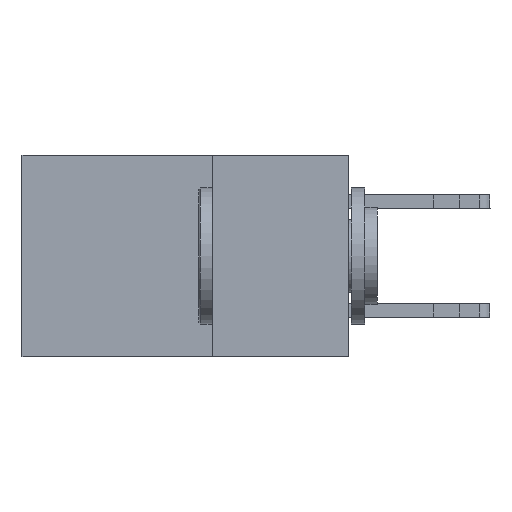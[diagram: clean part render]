
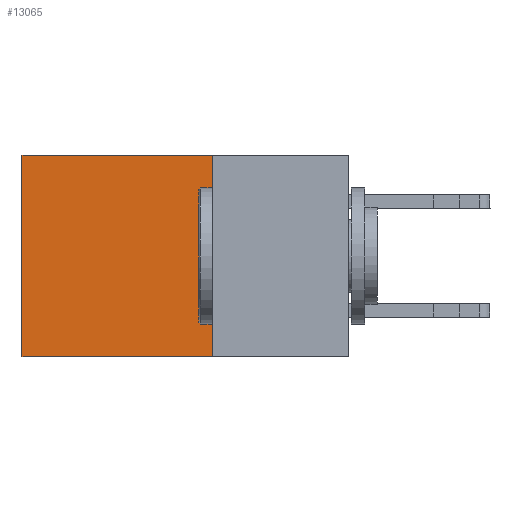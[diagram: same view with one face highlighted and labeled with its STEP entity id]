
A CAD part, left-side view. The second image highlights one B-rep face of the part: STEP entity #13065.
In plain terms, the highlighted planar face has unit normal (-1, 0, 0).
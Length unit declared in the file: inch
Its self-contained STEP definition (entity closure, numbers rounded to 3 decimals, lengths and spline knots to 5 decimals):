
#468 = DIRECTION ( 'NONE',  ( 1., 0., 0. ) ) ;
#1543 = LINE ( 'NONE', #2800, #16800 ) ;
#1731 = ORIENTED_EDGE ( 'NONE', *, *, #2839, .F. ) ;
#2800 = CARTESIAN_POINT ( 'NONE',  ( 0.2615, 0.25, 0. ) ) ;
#2839 = EDGE_CURVE ( 'NONE', #6203, #6541, #3443, .T. ) ;
#3443 = LINE ( 'NONE', #5105, #13022 ) ;
#3713 = LINE ( 'NONE', #8849, #19715 ) ;
#4498 = VERTEX_POINT ( 'NONE', #4589 ) ;
#4589 = CARTESIAN_POINT ( 'NONE',  ( 0.2615, 0.6, -0.37 ) ) ;
#4920 = VECTOR ( 'NONE', #8680, 39.37008 ) ;
#5105 = CARTESIAN_POINT ( 'NONE',  ( 0.2615, 0.25, -0.37 ) ) ;
#6203 = VERTEX_POINT ( 'NONE', #11312 ) ;
#6541 = VERTEX_POINT ( 'NONE', #18868 ) ;
#8680 = DIRECTION ( 'NONE',  ( 0., 1., 0. ) ) ;
#8849 = CARTESIAN_POINT ( 'NONE',  ( 0.2615, 0.6, -0.37 ) ) ;
#10042 = DIRECTION ( 'NONE',  ( 0., 0., -1. ) ) ;
#10146 = CARTESIAN_POINT ( 'NONE',  ( 0.2615, 0.25, -0.37 ) ) ;
#10993 = DIRECTION ( 'NONE',  ( 0., 1., 0. ) ) ;
#11118 = AXIS2_PLACEMENT_3D ( 'NONE', #14662, #468, #14451 ) ;
#11312 = CARTESIAN_POINT ( 'NONE',  ( 0.2615, 0.25, 0. ) ) ;
#11455 = FACE_OUTER_BOUND ( 'NONE', #13825, .T. ) ;
#12139 = ORIENTED_EDGE ( 'NONE', *, *, #17546, .T. ) ;
#12879 = DIRECTION ( 'NONE',  ( 0., 0., -1. ) ) ;
#13022 = VECTOR ( 'NONE', #12879, 39.37008 ) ;
#13065 = ADVANCED_FACE ( 'NONE', ( #11455 ), #17731, .F. ) ;
#13825 = EDGE_LOOP ( 'NONE', ( #14420, #18772, #1731, #12139 ) ) ;
#14217 = VERTEX_POINT ( 'NONE', #17322 ) ;
#14420 = ORIENTED_EDGE ( 'NONE', *, *, #15044, .T. ) ;
#14451 = DIRECTION ( 'NONE',  ( 0., 0., -1. ) ) ;
#14662 = CARTESIAN_POINT ( 'NONE',  ( 0.2615, 0.25, -0.37 ) ) ;
#15044 = EDGE_CURVE ( 'NONE', #14217, #4498, #3713, .T. ) ;
#16436 = LINE ( 'NONE', #10146, #4920 ) ;
#16470 = EDGE_CURVE ( 'NONE', #6541, #4498, #16436, .T. ) ;
#16800 = VECTOR ( 'NONE', #10993, 39.37008 ) ;
#17322 = CARTESIAN_POINT ( 'NONE',  ( 0.2615, 0.6, 0. ) ) ;
#17546 = EDGE_CURVE ( 'NONE', #6203, #14217, #1543, .T. ) ;
#17731 = PLANE ( 'NONE',  #11118 ) ;
#18772 = ORIENTED_EDGE ( 'NONE', *, *, #16470, .F. ) ;
#18868 = CARTESIAN_POINT ( 'NONE',  ( 0.2615, 0.25, -0.37 ) ) ;
#19715 = VECTOR ( 'NONE', #10042, 39.37008 ) ;
